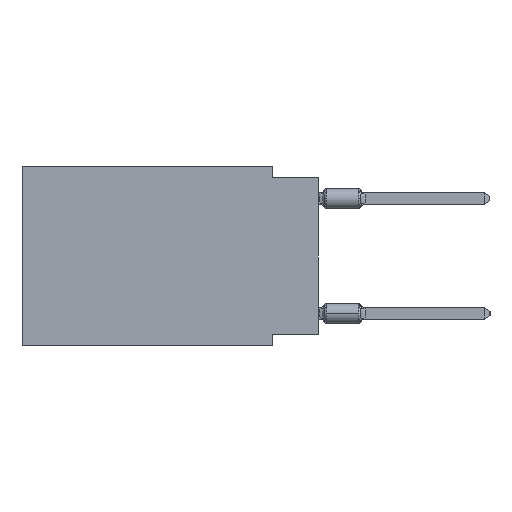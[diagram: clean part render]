
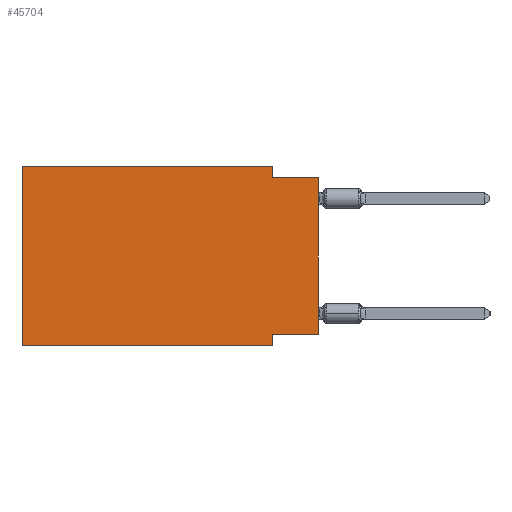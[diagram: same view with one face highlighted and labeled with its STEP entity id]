
A CAD part, left-side view. The second image highlights one B-rep face of the part: STEP entity #45704.
In plain terms, the highlighted planar face has unit normal (-1, 0, 0).
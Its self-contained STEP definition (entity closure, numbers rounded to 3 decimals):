
#411 = EDGE_LOOP ( 'NONE', ( #25381, #21080, #14243, #3692, #50461, #63383, #64907, #52559 ) ) ;
#897 = DIRECTION ( 'NONE',  ( 0., 0., -1. ) ) ;
#1279 = LINE ( 'NONE', #8212, #41226 ) ;
#2964 = VECTOR ( 'NONE', #46166, 1000. ) ;
#3692 = ORIENTED_EDGE ( 'NONE', *, *, #40867, .F. ) ;
#7847 = LINE ( 'NONE', #49057, #35494 ) ;
#7888 = AXIS2_PLACEMENT_3D ( 'NONE', #10622, #46798, #897 ) ;
#8212 = CARTESIAN_POINT ( 'NONE',  ( 0., 0., -9.271 ) ) ;
#10622 = CARTESIAN_POINT ( 'NONE',  ( 0., 16.383, 0. ) ) ;
#11408 = DIRECTION ( 'NONE',  ( 0., -1., 0. ) ) ;
#14243 = ORIENTED_EDGE ( 'NONE', *, *, #37305, .F. ) ;
#15107 = LINE ( 'NONE', #16101, #21187 ) ;
#15178 = VECTOR ( 'NONE', #11408, 1000. ) ;
#15397 = EDGE_CURVE ( 'NONE', #15493, #24785, #7847, .T. ) ;
#15493 = VERTEX_POINT ( 'NONE', #21152 ) ;
#15526 = EDGE_CURVE ( 'NONE', #49820, #24785, #31498, .T. ) ;
#16101 = CARTESIAN_POINT ( 'NONE',  ( 0., 0., -0.635 ) ) ;
#21080 = ORIENTED_EDGE ( 'NONE', *, *, #29981, .F. ) ;
#21152 = CARTESIAN_POINT ( 'NONE',  ( 0., 2.54, -9.271 ) ) ;
#21187 = VECTOR ( 'NONE', #26461, 1000. ) ;
#23299 = DIRECTION ( 'NONE',  ( 0., 1., 0. ) ) ;
#23410 = LINE ( 'NONE', #24053, #38701 ) ;
#24053 = CARTESIAN_POINT ( 'NONE',  ( 0., 0., 0. ) ) ;
#24785 = VERTEX_POINT ( 'NONE', #63627 ) ;
#25381 = ORIENTED_EDGE ( 'NONE', *, *, #42714, .T. ) ;
#25594 = CARTESIAN_POINT ( 'NONE',  ( 0., 0., -9.271 ) ) ;
#26461 = DIRECTION ( 'NONE',  ( 0., -1., 0. ) ) ;
#26492 = CARTESIAN_POINT ( 'NONE',  ( 0., 16.383, -9.906 ) ) ;
#29981 = EDGE_CURVE ( 'NONE', #66165, #33762, #15107, .T. ) ;
#31111 = CARTESIAN_POINT ( 'NONE',  ( 0., 16.383, -9.906 ) ) ;
#31498 = LINE ( 'NONE', #26492, #15178 ) ;
#33469 = DIRECTION ( 'NONE',  ( 0., 0., -1. ) ) ;
#33762 = VERTEX_POINT ( 'NONE', #42795 ) ;
#34448 = VERTEX_POINT ( 'NONE', #25594 ) ;
#34653 = CARTESIAN_POINT ( 'NONE',  ( 0., 16.383, 0. ) ) ;
#35494 = VECTOR ( 'NONE', #54078, 1000. ) ;
#36235 = LINE ( 'NONE', #55881, #2964 ) ;
#36581 = EDGE_CURVE ( 'NONE', #34448, #15493, #1279, .T. ) ;
#37305 = EDGE_CURVE ( 'NONE', #42094, #66165, #63291, .T. ) ;
#38701 = VECTOR ( 'NONE', #48509, 1000. ) ;
#38790 = VECTOR ( 'NONE', #55070, 1000. ) ;
#39957 = CARTESIAN_POINT ( 'NONE',  ( 0., 2.54, 0. ) ) ;
#40867 = EDGE_CURVE ( 'NONE', #60944, #42094, #36235, .T. ) ;
#41101 = PLANE ( 'NONE',  #7888 ) ;
#41226 = VECTOR ( 'NONE', #23299, 1000. ) ;
#41764 = FACE_OUTER_BOUND ( 'NONE', #411, .T. ) ;
#42094 = VERTEX_POINT ( 'NONE', #39957 ) ;
#42714 = EDGE_CURVE ( 'NONE', #34448, #33762, #23410, .T. ) ;
#42795 = CARTESIAN_POINT ( 'NONE',  ( 0., 0., -0.635 ) ) ;
#45704 = ADVANCED_FACE ( 'NONE', ( #41764 ), #41101, .F. ) ;
#46166 = DIRECTION ( 'NONE',  ( 0., -1., 0. ) ) ;
#46636 = VECTOR ( 'NONE', #33469, 1000. ) ;
#46798 = DIRECTION ( 'NONE',  ( 1., 0., 0. ) ) ;
#48509 = DIRECTION ( 'NONE',  ( 0., 0., 1. ) ) ;
#49057 = CARTESIAN_POINT ( 'NONE',  ( 0., 2.54, -9.906 ) ) ;
#49820 = VERTEX_POINT ( 'NONE', #31111 ) ;
#50461 = ORIENTED_EDGE ( 'NONE', *, *, #61752, .F. ) ;
#52559 = ORIENTED_EDGE ( 'NONE', *, *, #36581, .F. ) ;
#54078 = DIRECTION ( 'NONE',  ( 0., 0., -1. ) ) ;
#55070 = DIRECTION ( 'NONE',  ( 0., 0., 1. ) ) ;
#55881 = CARTESIAN_POINT ( 'NONE',  ( 0., 16.383, 0. ) ) ;
#59417 = CARTESIAN_POINT ( 'NONE',  ( 0., 2.54, -0.635 ) ) ;
#60944 = VERTEX_POINT ( 'NONE', #61494 ) ;
#61494 = CARTESIAN_POINT ( 'NONE',  ( 0., 16.383, 0. ) ) ;
#61752 = EDGE_CURVE ( 'NONE', #49820, #60944, #65128, .T. ) ;
#63291 = LINE ( 'NONE', #63618, #46636 ) ;
#63383 = ORIENTED_EDGE ( 'NONE', *, *, #15526, .T. ) ;
#63618 = CARTESIAN_POINT ( 'NONE',  ( 0., 2.54, 0. ) ) ;
#63627 = CARTESIAN_POINT ( 'NONE',  ( 0., 2.54, -9.906 ) ) ;
#64907 = ORIENTED_EDGE ( 'NONE', *, *, #15397, .F. ) ;
#65128 = LINE ( 'NONE', #34653, #38790 ) ;
#66165 = VERTEX_POINT ( 'NONE', #59417 ) ;
